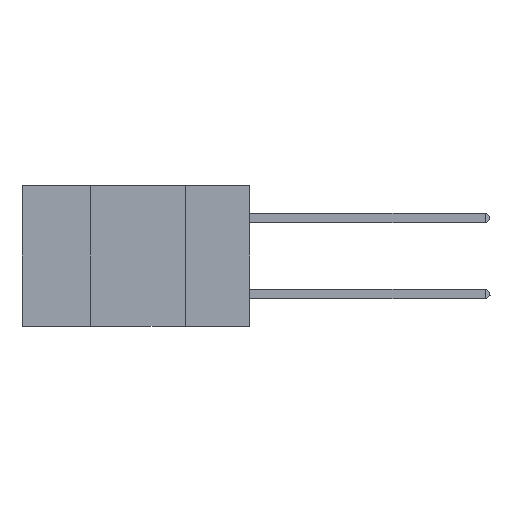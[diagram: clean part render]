
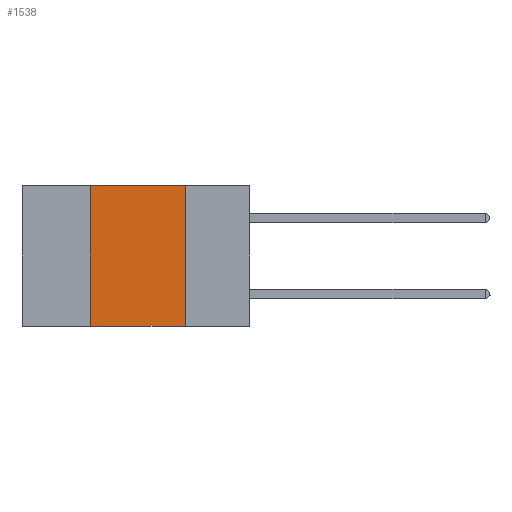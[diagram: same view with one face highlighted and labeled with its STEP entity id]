
A CAD part, left-side view. The second image highlights one B-rep face of the part: STEP entity #1538.
In plain terms, the highlighted planar face has unit normal (-1, 0, 0).
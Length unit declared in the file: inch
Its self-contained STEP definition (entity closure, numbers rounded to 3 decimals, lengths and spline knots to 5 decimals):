
#332 = CARTESIAN_POINT ( 'NONE',  ( 0., 0.42, 0. ) ) ;
#1504 = VERTEX_POINT ( 'NONE', #11989 ) ;
#1538 = ADVANCED_FACE ( 'NONE', ( #12226 ), #14319, .F. ) ;
#2423 = EDGE_CURVE ( 'NONE', #11556, #9977, #11472, .T. ) ;
#2759 = DIRECTION ( 'NONE',  ( 0., 0., -1. ) ) ;
#2895 = LINE ( 'NONE', #6657, #10781 ) ;
#4034 = CARTESIAN_POINT ( 'NONE',  ( 0., 0.6, 0. ) ) ;
#4134 = EDGE_CURVE ( 'NONE', #4397, #1504, #8538, .T. ) ;
#4397 = VERTEX_POINT ( 'NONE', #332 ) ;
#4559 = ORIENTED_EDGE ( 'NONE', *, *, #4134, .F. ) ;
#5413 = EDGE_LOOP ( 'NONE', ( #9875, #4559, #9773, #14172 ) ) ;
#5640 = DIRECTION ( 'NONE',  ( 0., 0., 1. ) ) ;
#5688 = EDGE_CURVE ( 'NONE', #1504, #9977, #8297, .T. ) ;
#6485 = EDGE_CURVE ( 'NONE', #11556, #4397, #2895, .T. ) ;
#6657 = CARTESIAN_POINT ( 'NONE',  ( 0., 0.42, 0. ) ) ;
#6932 = VECTOR ( 'NONE', #13628, 39.37008 ) ;
#7656 = CARTESIAN_POINT ( 'NONE',  ( 0., 0.17, 0. ) ) ;
#8297 = LINE ( 'NONE', #7656, #9195 ) ;
#8538 = LINE ( 'NONE', #8972, #6932 ) ;
#8616 = CARTESIAN_POINT ( 'NONE',  ( 0., 0.42, -0.37 ) ) ;
#8972 = CARTESIAN_POINT ( 'NONE',  ( 0., 0.6, 0. ) ) ;
#9195 = VECTOR ( 'NONE', #11092, 39.37008 ) ;
#9250 = CARTESIAN_POINT ( 'NONE',  ( 0., 0.6, -0.37 ) ) ;
#9301 = DIRECTION ( 'NONE',  ( 0., -1., 0. ) ) ;
#9773 = ORIENTED_EDGE ( 'NONE', *, *, #6485, .F. ) ;
#9875 = ORIENTED_EDGE ( 'NONE', *, *, #5688, .F. ) ;
#9977 = VERTEX_POINT ( 'NONE', #14166 ) ;
#10781 = VECTOR ( 'NONE', #5640, 39.37008 ) ;
#11092 = DIRECTION ( 'NONE',  ( 0., 0., -1. ) ) ;
#11472 = LINE ( 'NONE', #9250, #14353 ) ;
#11556 = VERTEX_POINT ( 'NONE', #8616 ) ;
#11989 = CARTESIAN_POINT ( 'NONE',  ( 0., 0.17, 0. ) ) ;
#12196 = AXIS2_PLACEMENT_3D ( 'NONE', #4034, #13261, #2759 ) ;
#12226 = FACE_OUTER_BOUND ( 'NONE', #5413, .T. ) ;
#13261 = DIRECTION ( 'NONE',  ( 1., 0., 0. ) ) ;
#13628 = DIRECTION ( 'NONE',  ( 0., -1., 0. ) ) ;
#14166 = CARTESIAN_POINT ( 'NONE',  ( 0., 0.17, -0.37 ) ) ;
#14172 = ORIENTED_EDGE ( 'NONE', *, *, #2423, .T. ) ;
#14319 = PLANE ( 'NONE',  #12196 ) ;
#14353 = VECTOR ( 'NONE', #9301, 39.37008 ) ;
